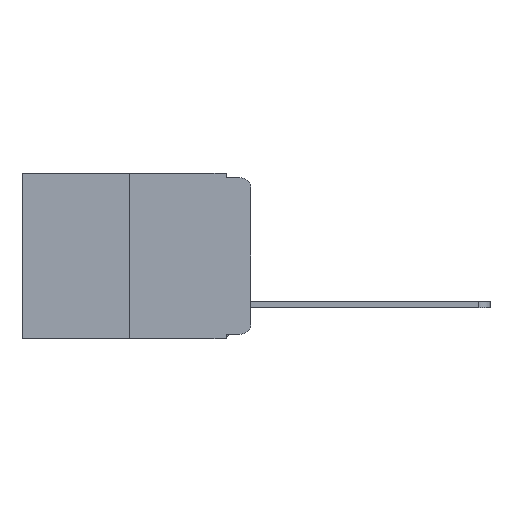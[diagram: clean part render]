
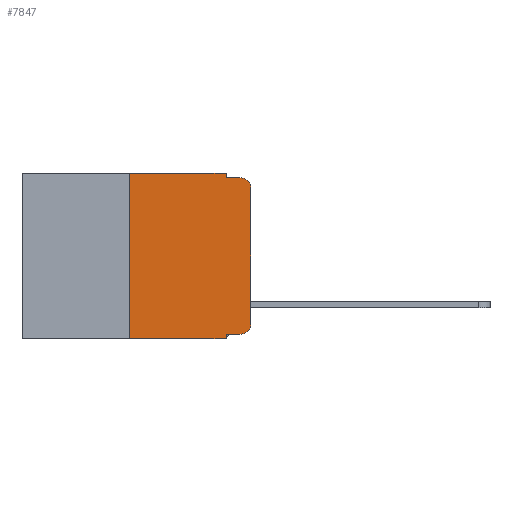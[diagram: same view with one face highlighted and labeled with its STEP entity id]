
A CAD part, left-side view. The second image highlights one B-rep face of the part: STEP entity #7847.
In plain terms, the highlighted planar face has unit normal (-1, 0, 0).
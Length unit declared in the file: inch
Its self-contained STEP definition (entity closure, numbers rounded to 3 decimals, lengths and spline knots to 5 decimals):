
#243 = VECTOR ( 'NONE', #18331, 39.37008 ) ;
#398 = DIRECTION ( 'NONE',  ( 0., 0., 1. ) ) ;
#853 = VECTOR ( 'NONE', #12822, 39.37008 ) ;
#892 = CARTESIAN_POINT ( 'NONE',  ( 0., 0.02, -0.333 ) ) ;
#950 = VERTEX_POINT ( 'NONE', #17121 ) ;
#989 = CARTESIAN_POINT ( 'NONE',  ( 0., 0.051, -0.01 ) ) ;
#1036 = AXIS2_PLACEMENT_3D ( 'NONE', #17976, #9193, #19321 ) ;
#1242 = PLANE ( 'NONE',  #11616 ) ;
#1244 = VECTOR ( 'NONE', #10076, 39.37008 ) ;
#1456 = ORIENTED_EDGE ( 'NONE', *, *, #10830, .T. ) ;
#1726 = FACE_OUTER_BOUND ( 'NONE', #5124, .T. ) ;
#2307 = LINE ( 'NONE', #11735, #1244 ) ;
#2454 = ORIENTED_EDGE ( 'NONE', *, *, #10355, .F. ) ;
#2670 = VERTEX_POINT ( 'NONE', #6307 ) ;
#2862 = AXIS2_PLACEMENT_3D ( 'NONE', #18381, #9688, #19731 ) ;
#3006 = DIRECTION ( 'NONE',  ( 1., 0., 0. ) ) ;
#3370 = VERTEX_POINT ( 'NONE', #16935 ) ;
#4253 = VERTEX_POINT ( 'NONE', #892 ) ;
#4283 = CARTESIAN_POINT ( 'NONE',  ( 0., 0.051, -0.333 ) ) ;
#5124 = EDGE_LOOP ( 'NONE', ( #9175, #14673, #7385, #18141, #2454, #5233, #1456, #16346, #14652, #19561 ) ) ;
#5233 = ORIENTED_EDGE ( 'NONE', *, *, #6692, .F. ) ;
#6062 = DIRECTION ( 'NONE',  ( 0., -1., 0. ) ) ;
#6307 = CARTESIAN_POINT ( 'NONE',  ( 0., 0.25, 0. ) ) ;
#6362 = CARTESIAN_POINT ( 'NONE',  ( 0., 0.25, -0.343 ) ) ;
#6613 = VERTEX_POINT ( 'NONE', #9807 ) ;
#6617 = VECTOR ( 'NONE', #398, 39.37008 ) ;
#6692 = EDGE_CURVE ( 'NONE', #16853, #2670, #6835, .T. ) ;
#6835 = LINE ( 'NONE', #10455, #10826 ) ;
#6910 = CARTESIAN_POINT ( 'NONE',  ( 0., 0.051, 0. ) ) ;
#7058 = DIRECTION ( 'NONE',  ( 0., 0., 1. ) ) ;
#7154 = LINE ( 'NONE', #17919, #6617 ) ;
#7283 = EDGE_CURVE ( 'NONE', #15902, #18744, #2307, .T. ) ;
#7385 = ORIENTED_EDGE ( 'NONE', *, *, #11144, .F. ) ;
#7444 = VECTOR ( 'NONE', #11404, 39.37008 ) ;
#7519 = LINE ( 'NONE', #4283, #15302 ) ;
#7529 = EDGE_CURVE ( 'NONE', #15902, #4253, #7519, .T. ) ;
#7586 = EDGE_CURVE ( 'NONE', #4253, #6613, #17620, .T. ) ;
#7841 = DIRECTION ( 'NONE',  ( 0., -1., 0. ) ) ;
#7847 = ADVANCED_FACE ( 'NONE', ( #1726 ), #1242, .F. ) ;
#8044 = CARTESIAN_POINT ( 'NONE',  ( 0., 0.473, -0.343 ) ) ;
#8288 = VECTOR ( 'NONE', #7841, 39.37008 ) ;
#9175 = ORIENTED_EDGE ( 'NONE', *, *, #11111, .T. ) ;
#9193 = DIRECTION ( 'NONE',  ( -1., 0., 0. ) ) ;
#9632 = CARTESIAN_POINT ( 'NONE',  ( 0., 0.051, 0. ) ) ;
#9688 = DIRECTION ( 'NONE',  ( -1., 0., 0. ) ) ;
#9807 = CARTESIAN_POINT ( 'NONE',  ( 0., 0., -0.313 ) ) ;
#9873 = CARTESIAN_POINT ( 'NONE',  ( 0., 0.473, 0. ) ) ;
#10076 = DIRECTION ( 'NONE',  ( 0., 0., -1. ) ) ;
#10355 = EDGE_CURVE ( 'NONE', #2670, #19142, #19917, .T. ) ;
#10455 = CARTESIAN_POINT ( 'NONE',  ( 0., 0.25, 0. ) ) ;
#10826 = VECTOR ( 'NONE', #7058, 39.37008 ) ;
#10830 = EDGE_CURVE ( 'NONE', #16853, #18744, #19250, .T. ) ;
#11111 = EDGE_CURVE ( 'NONE', #6613, #15978, #7154, .T. ) ;
#11113 = EDGE_CURVE ( 'NONE', #15978, #950, #11623, .T. ) ;
#11144 = EDGE_CURVE ( 'NONE', #3370, #950, #17344, .T. ) ;
#11150 = EDGE_CURVE ( 'NONE', #19142, #3370, #14548, .T. ) ;
#11404 = DIRECTION ( 'NONE',  ( 0., -1., 0. ) ) ;
#11616 = AXIS2_PLACEMENT_3D ( 'NONE', #9873, #3006, #14453 ) ;
#11623 = CIRCLE ( 'NONE', #1036, 0.02 ) ;
#11735 = CARTESIAN_POINT ( 'NONE',  ( 0., 0.051, 0. ) ) ;
#12822 = DIRECTION ( 'NONE',  ( 0., -1., 0. ) ) ;
#14453 = DIRECTION ( 'NONE',  ( 0., 0., -1. ) ) ;
#14467 = CARTESIAN_POINT ( 'NONE',  ( 0., 0.051, -0.343 ) ) ;
#14548 = LINE ( 'NONE', #9632, #243 ) ;
#14652 = ORIENTED_EDGE ( 'NONE', *, *, #7529, .T. ) ;
#14673 = ORIENTED_EDGE ( 'NONE', *, *, #11113, .T. ) ;
#14917 = CARTESIAN_POINT ( 'NONE',  ( 0., 0., -0.03 ) ) ;
#15302 = VECTOR ( 'NONE', #6062, 39.37008 ) ;
#15902 = VERTEX_POINT ( 'NONE', #18958 ) ;
#15978 = VERTEX_POINT ( 'NONE', #14917 ) ;
#16346 = ORIENTED_EDGE ( 'NONE', *, *, #7283, .F. ) ;
#16838 = CARTESIAN_POINT ( 'NONE',  ( 0., 0.473, 0. ) ) ;
#16853 = VERTEX_POINT ( 'NONE', #6362 ) ;
#16935 = CARTESIAN_POINT ( 'NONE',  ( 0., 0.051, -0.01 ) ) ;
#17121 = CARTESIAN_POINT ( 'NONE',  ( 0., 0.02, -0.01 ) ) ;
#17344 = LINE ( 'NONE', #989, #853 ) ;
#17620 = CIRCLE ( 'NONE', #2862, 0.02 ) ;
#17919 = CARTESIAN_POINT ( 'NONE',  ( 0., 0., 0. ) ) ;
#17976 = CARTESIAN_POINT ( 'NONE',  ( 0., 0.02, -0.03 ) ) ;
#18141 = ORIENTED_EDGE ( 'NONE', *, *, #11150, .F. ) ;
#18331 = DIRECTION ( 'NONE',  ( 0., 0., -1. ) ) ;
#18381 = CARTESIAN_POINT ( 'NONE',  ( 0., 0.02, -0.313 ) ) ;
#18744 = VERTEX_POINT ( 'NONE', #14467 ) ;
#18958 = CARTESIAN_POINT ( 'NONE',  ( 0., 0.051, -0.333 ) ) ;
#19142 = VERTEX_POINT ( 'NONE', #6910 ) ;
#19250 = LINE ( 'NONE', #8044, #7444 ) ;
#19321 = DIRECTION ( 'NONE',  ( 0., 0., -1. ) ) ;
#19561 = ORIENTED_EDGE ( 'NONE', *, *, #7586, .T. ) ;
#19731 = DIRECTION ( 'NONE',  ( 0., 0., -1. ) ) ;
#19917 = LINE ( 'NONE', #16838, #8288 ) ;
